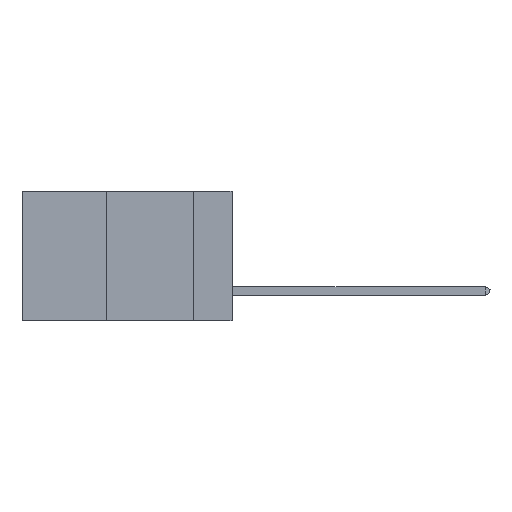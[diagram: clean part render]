
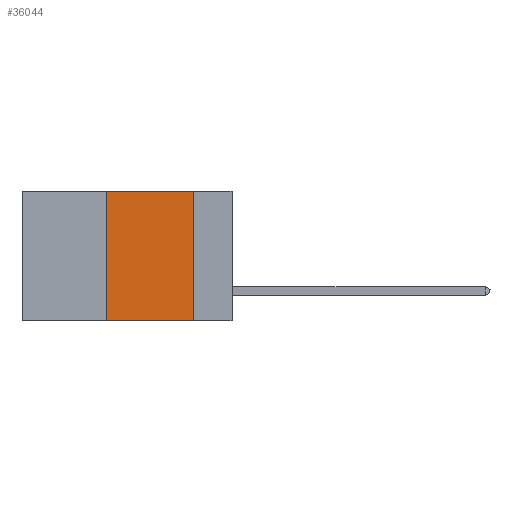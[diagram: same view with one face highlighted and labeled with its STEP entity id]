
A CAD part, left-side view. The second image highlights one B-rep face of the part: STEP entity #36044.
In plain terms, the highlighted planar face has unit normal (-1, 0, 0).
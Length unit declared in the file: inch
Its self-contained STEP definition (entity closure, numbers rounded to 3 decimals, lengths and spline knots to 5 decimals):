
#1351 = EDGE_CURVE ( 'NONE', #2100, #42521, #23044, .T. ) ;
#2100 = VERTEX_POINT ( 'NONE', #27549 ) ;
#2190 = PLANE ( 'NONE',  #8427 ) ;
#3691 = VECTOR ( 'NONE', #48204, 39.37008 ) ;
#6948 = DIRECTION ( 'NONE',  ( 0., 0., 1. ) ) ;
#6965 = FACE_OUTER_BOUND ( 'NONE', #39878, .T. ) ;
#7248 = CARTESIAN_POINT ( 'NONE',  ( 0., 0.6, -0.37 ) ) ;
#8427 = AXIS2_PLACEMENT_3D ( 'NONE', #31779, #20572, #17284 ) ;
#12789 = CARTESIAN_POINT ( 'NONE',  ( 0., 0.11, 0. ) ) ;
#13397 = LINE ( 'NONE', #23260, #42845 ) ;
#17284 = DIRECTION ( 'NONE',  ( 0., 0., -1. ) ) ;
#19094 = LINE ( 'NONE', #7248, #3691 ) ;
#19912 = ORIENTED_EDGE ( 'NONE', *, *, #22497, .F. ) ;
#20572 = DIRECTION ( 'NONE',  ( 1., 0., 0. ) ) ;
#22058 = CARTESIAN_POINT ( 'NONE',  ( 0., 0.36, 0. ) ) ;
#22386 = ORIENTED_EDGE ( 'NONE', *, *, #1351, .F. ) ;
#22497 = EDGE_CURVE ( 'NONE', #46361, #23324, #41999, .T. ) ;
#23044 = LINE ( 'NONE', #12789, #24236 ) ;
#23260 = CARTESIAN_POINT ( 'NONE',  ( 0., 0.6, 0. ) ) ;
#23324 = VERTEX_POINT ( 'NONE', #30622 ) ;
#24236 = VECTOR ( 'NONE', #46723, 39.37008 ) ;
#24356 = VECTOR ( 'NONE', #6948, 39.37008 ) ;
#27549 = CARTESIAN_POINT ( 'NONE',  ( 0., 0.11, 0. ) ) ;
#30622 = CARTESIAN_POINT ( 'NONE',  ( 0., 0.36, 0. ) ) ;
#30869 = ORIENTED_EDGE ( 'NONE', *, *, #45861, .F. ) ;
#31779 = CARTESIAN_POINT ( 'NONE',  ( 0., 0.6, 0. ) ) ;
#36044 = ADVANCED_FACE ( 'NONE', ( #6965 ), #2190, .F. ) ;
#38420 = CARTESIAN_POINT ( 'NONE',  ( 0., 0.36, -0.37 ) ) ;
#39774 = EDGE_CURVE ( 'NONE', #46361, #42521, #19094, .T. ) ;
#39878 = EDGE_LOOP ( 'NONE', ( #22386, #30869, #19912, #44633 ) ) ;
#41700 = DIRECTION ( 'NONE',  ( 0., -1., 0. ) ) ;
#41871 = CARTESIAN_POINT ( 'NONE',  ( 0., 0.11, -0.37 ) ) ;
#41999 = LINE ( 'NONE', #22058, #24356 ) ;
#42521 = VERTEX_POINT ( 'NONE', #41871 ) ;
#42845 = VECTOR ( 'NONE', #41700, 39.37008 ) ;
#44633 = ORIENTED_EDGE ( 'NONE', *, *, #39774, .T. ) ;
#45861 = EDGE_CURVE ( 'NONE', #23324, #2100, #13397, .T. ) ;
#46361 = VERTEX_POINT ( 'NONE', #38420 ) ;
#46723 = DIRECTION ( 'NONE',  ( 0., 0., -1. ) ) ;
#48204 = DIRECTION ( 'NONE',  ( 0., -1., 0. ) ) ;
